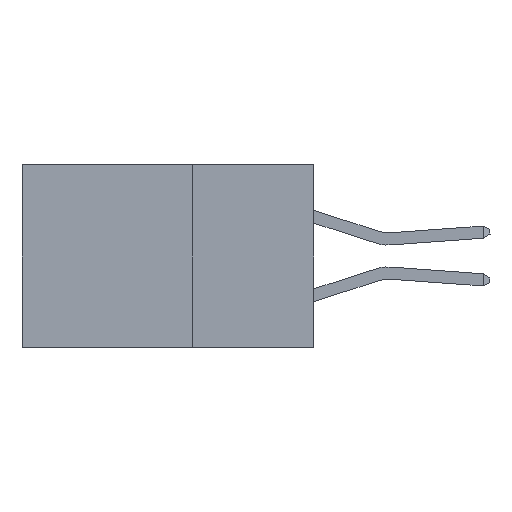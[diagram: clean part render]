
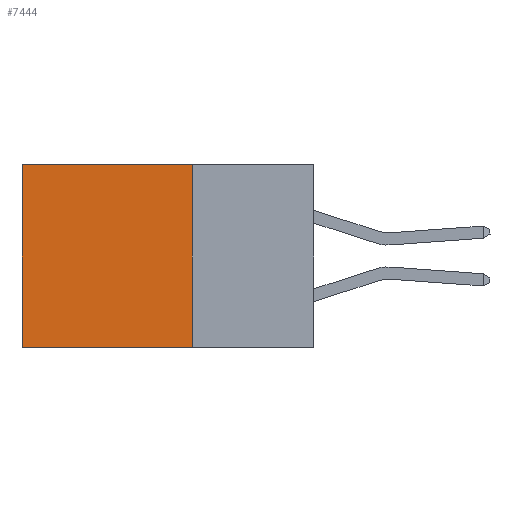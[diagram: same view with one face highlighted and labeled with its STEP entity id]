
A CAD part, left-side view. The second image highlights one B-rep face of the part: STEP entity #7444.
In plain terms, the highlighted planar face has unit normal (-1, 0, 0).
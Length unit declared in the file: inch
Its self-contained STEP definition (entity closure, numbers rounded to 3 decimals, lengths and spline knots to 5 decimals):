
#75 = DIRECTION ( 'NONE',  ( 0., 0., -1. ) ) ;
#497 = CARTESIAN_POINT ( 'NONE',  ( 0.2875, 0.25, -0.375 ) ) ;
#686 = CARTESIAN_POINT ( 'NONE',  ( 0.2875, 0.25, 0. ) ) ;
#1154 = LINE ( 'NONE', #2322, #1875 ) ;
#1240 = AXIS2_PLACEMENT_3D ( 'NONE', #5716, #4970, #4232 ) ;
#1333 = VERTEX_POINT ( 'NONE', #686 ) ;
#1636 = VECTOR ( 'NONE', #75, 39.37008 ) ;
#1796 = LINE ( 'NONE', #2147, #7070 ) ;
#1875 = VECTOR ( 'NONE', #6851, 39.37008 ) ;
#2147 = CARTESIAN_POINT ( 'NONE',  ( 0.2875, 0.6, -0.375 ) ) ;
#2322 = CARTESIAN_POINT ( 'NONE',  ( 0.2875, 0.25, 0. ) ) ;
#2439 = VERTEX_POINT ( 'NONE', #8266 ) ;
#2612 = EDGE_CURVE ( 'NONE', #1333, #9680, #6655, .T. ) ;
#3428 = PLANE ( 'NONE',  #1240 ) ;
#3714 = EDGE_CURVE ( 'NONE', #1333, #5067, #1154, .T. ) ;
#3991 = ORIENTED_EDGE ( 'NONE', *, *, #9650, .T. ) ;
#4208 = FACE_OUTER_BOUND ( 'NONE', #5223, .T. ) ;
#4232 = DIRECTION ( 'NONE',  ( 0., 0., -1. ) ) ;
#4472 = LINE ( 'NONE', #497, #5927 ) ;
#4905 = ORIENTED_EDGE ( 'NONE', *, *, #6255, .F. ) ;
#4970 = DIRECTION ( 'NONE',  ( 1., 0., 0. ) ) ;
#5067 = VERTEX_POINT ( 'NONE', #6502 ) ;
#5223 = EDGE_LOOP ( 'NONE', ( #3991, #4905, #7855, #7297 ) ) ;
#5716 = CARTESIAN_POINT ( 'NONE',  ( 0.2875, 0.25, -0.375 ) ) ;
#5927 = VECTOR ( 'NONE', #7341, 39.37008 ) ;
#6191 = CARTESIAN_POINT ( 'NONE',  ( 0.2875, 0.25, -0.375 ) ) ;
#6255 = EDGE_CURVE ( 'NONE', #9680, #2439, #4472, .T. ) ;
#6502 = CARTESIAN_POINT ( 'NONE',  ( 0.2875, 0.6, 0. ) ) ;
#6655 = LINE ( 'NONE', #7052, #1636 ) ;
#6851 = DIRECTION ( 'NONE',  ( 0., 1., 0. ) ) ;
#7052 = CARTESIAN_POINT ( 'NONE',  ( 0.2875, 0.25, -0.375 ) ) ;
#7070 = VECTOR ( 'NONE', #8260, 39.37008 ) ;
#7297 = ORIENTED_EDGE ( 'NONE', *, *, #3714, .T. ) ;
#7341 = DIRECTION ( 'NONE',  ( 0., 1., 0. ) ) ;
#7444 = ADVANCED_FACE ( 'NONE', ( #4208 ), #3428, .F. ) ;
#7855 = ORIENTED_EDGE ( 'NONE', *, *, #2612, .F. ) ;
#8260 = DIRECTION ( 'NONE',  ( 0., 0., -1. ) ) ;
#8266 = CARTESIAN_POINT ( 'NONE',  ( 0.2875, 0.6, -0.375 ) ) ;
#9650 = EDGE_CURVE ( 'NONE', #5067, #2439, #1796, .T. ) ;
#9680 = VERTEX_POINT ( 'NONE', #6191 ) ;
